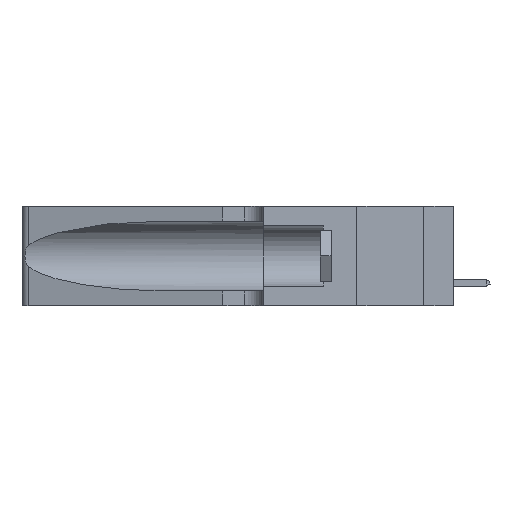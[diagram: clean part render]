
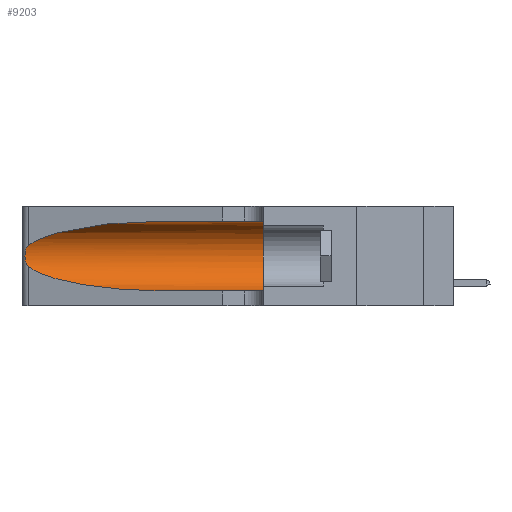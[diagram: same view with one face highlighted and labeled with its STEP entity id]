
A CAD part, left-side view. The second image highlights one B-rep face of the part: STEP entity #9203.
In plain terms, the highlighted cylindrical face has radius 3.308 mm (diameter 6.617 mm), a partial arc.
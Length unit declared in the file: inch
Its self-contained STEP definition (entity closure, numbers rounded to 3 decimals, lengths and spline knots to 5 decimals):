
#207 = CARTESIAN_POINT ( 'NONE',  ( 0.1305, 0.35, 0.185 ) ) ;
#952 = ORIENTED_EDGE ( 'NONE', *, *, #13805, .F. ) ;
#1569 = EDGE_LOOP ( 'NONE', ( #33138, #24053, #44775, #9289, #952, #41395 ) ) ;
#2746 = EDGE_CURVE ( 'NONE', #7228, #2851, #12080, .T. ) ;
#2851 = VERTEX_POINT ( 'NONE', #30012 ) ;
#3597 = CARTESIAN_POINT ( 'NONE',  ( 0.18966, 0.96281, 0.31525 ) ) ;
#3623 = CARTESIAN_POINT ( 'NONE',  ( 0.25856, 1.23593, 0.16098 ) ) ;
#3943 = EDGE_CURVE ( 'NONE', #36777, #4116, #25240, .T. ) ;
#4116 = VERTEX_POINT ( 'NONE', #45441 ) ;
#7228 = VERTEX_POINT ( 'NONE', #16456 ) ;
#7414 = CARTESIAN_POINT ( 'NONE',  ( 0.25487, 1.22718, 0.22369 ) ) ;
#7746 = CARTESIAN_POINT ( 'NONE',  ( 0.25789, 1.23486, 0.15765 ) ) ;
#8722 = CARTESIAN_POINT ( 'NONE',  ( 0.25487, 1.22718, 0.22369 ) ) ;
#9068 = DIRECTION ( 'NONE',  ( 0., 1., 0. ) ) ;
#9203 = ADVANCED_FACE ( 'NONE', ( #37728 ), #45648, .F. ) ;
#9289 = ORIENTED_EDGE ( 'NONE', *, *, #24223, .T. ) ;
#11352 = CARTESIAN_POINT ( 'NONE',  ( 0.25555, 1.22994, 0.2215 ) ) ;
#12080 = LINE ( 'NONE', #33597, #28564 ) ;
#13419 = CARTESIAN_POINT ( 'NONE',  ( 0.25487, 1.22718, 0.14631 ) ) ;
#13805 = EDGE_CURVE ( 'NONE', #2851, #33683, #25289, .T. ) ;
#13969 = EDGE_CURVE ( 'NONE', #7228, #46736, #19930, .T. ) ;
#16112 = CARTESIAN_POINT ( 'NONE',  ( 0.25487, 1.22718, 0.22369 ) ) ;
#16456 = CARTESIAN_POINT ( 'NONE',  ( 0.1305, 0.72297, 0.31525 ) ) ;
#16758 = DIRECTION ( 'NONE',  ( 0., 0., 1. ) ) ;
#18185 = DIRECTION ( 'NONE',  ( 0., 0., -1. ) ) ;
#18999 = CARTESIAN_POINT ( 'NONE',  ( 0.25854, 1.2359, 0.20912 ) ) ;
#19202 = CARTESIAN_POINT ( 'NONE',  ( 0.1305, 0.35, 0.05475 ) ) ;
#19930 =( BOUNDED_CURVE ( )  B_SPLINE_CURVE ( 3, ( #23070, #3597, #31595, #8722 ),
 .UNSPECIFIED., .F., .F. ) 
 B_SPLINE_CURVE_WITH_KNOTS ( ( 4, 4 ),
 ( 1.5708, 2.84003 ),
 .UNSPECIFIED. ) 
 CURVE ( )  GEOMETRIC_REPRESENTATION_ITEM ( )  RATIONAL_B_SPLINE_CURVE ( ( 1., 0.87, 0.87, 1. ) ) 
 REPRESENTATION_ITEM ( '' )  );
#21800 = EDGE_CURVE ( 'NONE', #46736, #36777, #26191, .T. ) ;
#23070 = CARTESIAN_POINT ( 'NONE',  ( 0.1305, 0.72297, 0.31525 ) ) ;
#23443 = CARTESIAN_POINT ( 'NONE',  ( 0.26075, 1.23896, 0.178 ) ) ;
#24053 = ORIENTED_EDGE ( 'NONE', *, *, #21800, .T. ) ;
#24223 = EDGE_CURVE ( 'NONE', #4116, #33683, #39104, .T. ) ;
#25240 =( BOUNDED_CURVE ( )  B_SPLINE_CURVE ( 3, ( #36427, #25322, #25493, #44595 ),
 .UNSPECIFIED., .F., .F. ) 
 B_SPLINE_CURVE_WITH_KNOTS ( ( 4, 4 ),
 ( 3.44316, 4.71239 ),
 .UNSPECIFIED. ) 
 CURVE ( )  GEOMETRIC_REPRESENTATION_ITEM ( )  RATIONAL_B_SPLINE_CURVE ( ( 1., 0.87, 0.87, 1. ) ) 
 REPRESENTATION_ITEM ( '' )  );
#25289 = CIRCLE ( 'NONE', #26842, 0.13025 ) ;
#25322 = CARTESIAN_POINT ( 'NONE',  ( 0.2373, 1.15595, 0.08982 ) ) ;
#25493 = CARTESIAN_POINT ( 'NONE',  ( 0.18966, 0.96281, 0.05475 ) ) ;
#26191 = B_SPLINE_CURVE_WITH_KNOTS ( 'NONE', 3,
 ( #7414, #11352, #27211, #46501, #18999, #31139, #27044, #23443, #35210, #3623, #7746, #47004, #31305, #35039 ),
 .UNSPECIFIED., .F., .F.,
 ( 4, 2, 2, 2, 2, 2, 4 ),
 ( 0., 0.00027, 0.00053, 0.00107, 0.0016, 0.00187, 0.00214 ),
 .UNSPECIFIED. ) ;
#26781 = DIRECTION ( 'NONE',  ( 0., -1., 0. ) ) ;
#26842 = AXIS2_PLACEMENT_3D ( 'NONE', #207, #9068, #16758 ) ;
#27044 = CARTESIAN_POINT ( 'NONE',  ( 0.26075, 1.23896, 0.19203 ) ) ;
#27211 = CARTESIAN_POINT ( 'NONE',  ( 0.25639, 1.23184, 0.21858 ) ) ;
#27472 = CARTESIAN_POINT ( 'NONE',  ( 0.1305, 1.61858, 0.05475 ) ) ;
#28564 = VECTOR ( 'NONE', #48949, 39.37008 ) ;
#30012 = CARTESIAN_POINT ( 'NONE',  ( 0.1305, 0.35, 0.31525 ) ) ;
#31139 = CARTESIAN_POINT ( 'NONE',  ( 0.26018, 1.23835, 0.19895 ) ) ;
#31305 = CARTESIAN_POINT ( 'NONE',  ( 0.25555, 1.22993, 0.14849 ) ) ;
#31595 = CARTESIAN_POINT ( 'NONE',  ( 0.2373, 1.15595, 0.28018 ) ) ;
#33138 = ORIENTED_EDGE ( 'NONE', *, *, #13969, .T. ) ;
#33597 = CARTESIAN_POINT ( 'NONE',  ( 0.1305, 1.61858, 0.31525 ) ) ;
#33683 = VERTEX_POINT ( 'NONE', #19202 ) ;
#35039 = CARTESIAN_POINT ( 'NONE',  ( 0.25487, 1.22718, 0.14631 ) ) ;
#35188 = AXIS2_PLACEMENT_3D ( 'NONE', #41580, #38002, #18185 ) ;
#35210 = CARTESIAN_POINT ( 'NONE',  ( 0.26017, 1.23833, 0.17102 ) ) ;
#36427 = CARTESIAN_POINT ( 'NONE',  ( 0.25487, 1.22718, 0.14631 ) ) ;
#36777 = VERTEX_POINT ( 'NONE', #13419 ) ;
#37728 = FACE_OUTER_BOUND ( 'NONE', #1569, .T. ) ;
#37875 = VECTOR ( 'NONE', #26781, 39.37008 ) ;
#38002 = DIRECTION ( 'NONE',  ( 0., -1., 0. ) ) ;
#39104 = LINE ( 'NONE', #27472, #37875 ) ;
#41395 = ORIENTED_EDGE ( 'NONE', *, *, #2746, .F. ) ;
#41580 = CARTESIAN_POINT ( 'NONE',  ( 0.1305, 1.61858, 0.185 ) ) ;
#44595 = CARTESIAN_POINT ( 'NONE',  ( 0.1305, 0.72297, 0.05475 ) ) ;
#44775 = ORIENTED_EDGE ( 'NONE', *, *, #3943, .T. ) ;
#45441 = CARTESIAN_POINT ( 'NONE',  ( 0.1305, 0.72297, 0.05475 ) ) ;
#45648 = CYLINDRICAL_SURFACE ( 'NONE', #35188, 0.13025 ) ;
#46501 = CARTESIAN_POINT ( 'NONE',  ( 0.25787, 1.23484, 0.2124 ) ) ;
#46736 = VERTEX_POINT ( 'NONE', #16112 ) ;
#47004 = CARTESIAN_POINT ( 'NONE',  ( 0.25639, 1.23186, 0.15144 ) ) ;
#48949 = DIRECTION ( 'NONE',  ( 0., -1., 0. ) ) ;
